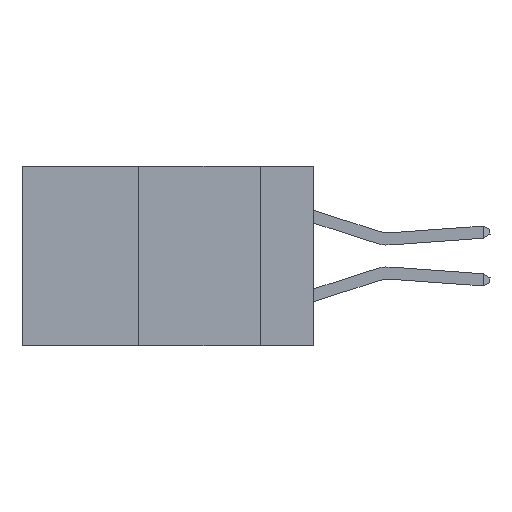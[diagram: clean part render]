
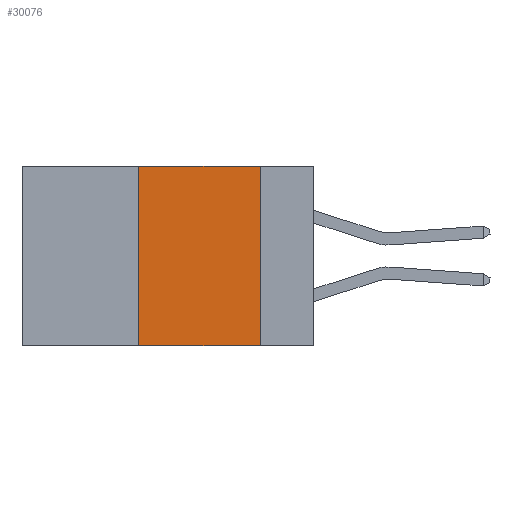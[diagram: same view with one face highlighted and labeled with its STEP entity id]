
A CAD part, left-side view. The second image highlights one B-rep face of the part: STEP entity #30076.
In plain terms, the highlighted planar face has unit normal (-1, 0, 0).
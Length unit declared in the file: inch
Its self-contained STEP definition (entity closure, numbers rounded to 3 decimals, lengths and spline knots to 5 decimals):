
#1079 = DIRECTION ( 'NONE',  ( 0., 0., -1. ) ) ;
#1425 = DIRECTION ( 'NONE',  ( 0., -1., 0. ) ) ;
#2056 = VECTOR ( 'NONE', #1425, 39.37008 ) ;
#2095 = DIRECTION ( 'NONE',  ( 0., -1., 0. ) ) ;
#2378 = EDGE_CURVE ( 'NONE', #28699, #25794, #19482, .T. ) ;
#2841 = LINE ( 'NONE', #21091, #2056 ) ;
#3465 = VECTOR ( 'NONE', #9492, 39.37008 ) ;
#4655 = ORIENTED_EDGE ( 'NONE', *, *, #22748, .F. ) ;
#4850 = VECTOR ( 'NONE', #2095, 39.37008 ) ;
#5312 = CARTESIAN_POINT ( 'NONE',  ( 0., 0.36, -0.37 ) ) ;
#5413 = ORIENTED_EDGE ( 'NONE', *, *, #6156, .F. ) ;
#6156 = EDGE_CURVE ( 'NONE', #25794, #17039, #26632, .T. ) ;
#6993 = CARTESIAN_POINT ( 'NONE',  ( 0., 0.36, 0. ) ) ;
#7311 = VECTOR ( 'NONE', #10283, 39.37008 ) ;
#8106 = ORIENTED_EDGE ( 'NONE', *, *, #27664, .T. ) ;
#9492 = DIRECTION ( 'NONE',  ( 0., 0., 1. ) ) ;
#9601 = EDGE_LOOP ( 'NONE', ( #5413, #16593, #4655, #8106 ) ) ;
#9991 = LINE ( 'NONE', #6993, #3465 ) ;
#10283 = DIRECTION ( 'NONE',  ( 0., 0., -1. ) ) ;
#10977 = VERTEX_POINT ( 'NONE', #5312 ) ;
#12177 = CARTESIAN_POINT ( 'NONE',  ( 0., 0.11, 0. ) ) ;
#13358 = CARTESIAN_POINT ( 'NONE',  ( 0., 0.6, 0. ) ) ;
#15835 = DIRECTION ( 'NONE',  ( 1., 0., 0. ) ) ;
#16593 = ORIENTED_EDGE ( 'NONE', *, *, #2378, .F. ) ;
#17039 = VERTEX_POINT ( 'NONE', #19366 ) ;
#19366 = CARTESIAN_POINT ( 'NONE',  ( 0., 0.11, -0.37 ) ) ;
#19482 = LINE ( 'NONE', #22267, #4850 ) ;
#21091 = CARTESIAN_POINT ( 'NONE',  ( 0., 0.6, -0.37 ) ) ;
#22267 = CARTESIAN_POINT ( 'NONE',  ( 0., 0.6, 0. ) ) ;
#22748 = EDGE_CURVE ( 'NONE', #10977, #28699, #9991, .T. ) ;
#23560 = FACE_OUTER_BOUND ( 'NONE', #9601, .T. ) ;
#24793 = CARTESIAN_POINT ( 'NONE',  ( 0., 0.36, 0. ) ) ;
#24876 = AXIS2_PLACEMENT_3D ( 'NONE', #13358, #15835, #1079 ) ;
#25794 = VERTEX_POINT ( 'NONE', #12177 ) ;
#26632 = LINE ( 'NONE', #29338, #7311 ) ;
#27657 = PLANE ( 'NONE',  #24876 ) ;
#27664 = EDGE_CURVE ( 'NONE', #10977, #17039, #2841, .T. ) ;
#28699 = VERTEX_POINT ( 'NONE', #24793 ) ;
#29338 = CARTESIAN_POINT ( 'NONE',  ( 0., 0.11, 0. ) ) ;
#30076 = ADVANCED_FACE ( 'NONE', ( #23560 ), #27657, .F. ) ;
